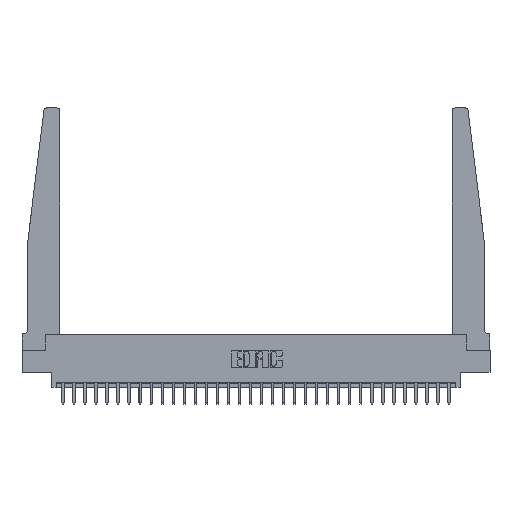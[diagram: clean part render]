
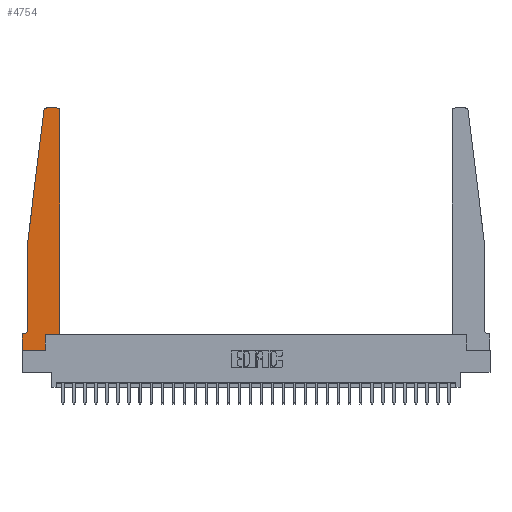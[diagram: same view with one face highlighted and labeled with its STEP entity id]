
A CAD part, top view. The second image highlights one B-rep face of the part: STEP entity #4754.
In plain terms, the highlighted planar face has unit normal (0, 0, 1).
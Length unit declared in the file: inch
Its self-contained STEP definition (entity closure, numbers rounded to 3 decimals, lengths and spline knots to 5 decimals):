
#468 = DIRECTION ( 'NONE',  ( 1., 0., 0. ) ) ;
#933 = CARTESIAN_POINT ( 'NONE',  ( 0., 0.1875, 0.37 ) ) ;
#1114 = DIRECTION ( 'NONE',  ( 0., -1., 0. ) ) ;
#1173 = VERTEX_POINT ( 'NONE', #16668 ) ;
#1797 = CARTESIAN_POINT ( 'NONE',  ( 0.015, 0.2375, 0.37 ) ) ;
#1874 = DIRECTION ( 'NONE',  ( 1., 0., 0. ) ) ;
#1889 = DIRECTION ( 'NONE',  ( 0., 0., 1. ) ) ;
#1945 = AXIS2_PLACEMENT_3D ( 'NONE', #16407, #14240, #468 ) ;
#2055 = DIRECTION ( 'NONE',  ( 0., 0., 1. ) ) ;
#2210 = CARTESIAN_POINT ( 'NONE',  ( 0.395, 2.72, 0.37 ) ) ;
#2400 = VERTEX_POINT ( 'NONE', #8629 ) ;
#2438 = DIRECTION ( 'NONE',  ( -0.122, -0.992, 0. ) ) ;
#2658 = ORIENTED_EDGE ( 'NONE', *, *, #6890, .T. ) ;
#2750 = VERTEX_POINT ( 'NONE', #17528 ) ;
#3119 = EDGE_CURVE ( 'NONE', #2400, #12083, #6324, .T. ) ;
#3208 = VECTOR ( 'NONE', #19406, 39.37008 ) ;
#4072 = DIRECTION ( 'NONE',  ( -1., 0., 0. ) ) ;
#4400 = VERTEX_POINT ( 'NONE', #13147 ) ;
#4754 = ADVANCED_FACE ( 'NONE', ( #12730 ), #25433, .T. ) ;
#5271 = CARTESIAN_POINT ( 'NONE',  ( 0.425, 0.18, 0.37 ) ) ;
#5695 = CARTESIAN_POINT ( 'NONE',  ( 0., 0., 0.37 ) ) ;
#6026 = EDGE_CURVE ( 'NONE', #26248, #22530, #23623, .T. ) ;
#6082 = CARTESIAN_POINT ( 'NONE',  ( 0.27653, 2.75, 0.37 ) ) ;
#6324 = CIRCLE ( 'NONE', #12543, 0.03 ) ;
#6637 = EDGE_CURVE ( 'NONE', #16781, #18427, #27081, .T. ) ;
#6890 = EDGE_CURVE ( 'NONE', #18427, #2750, #14757, .T. ) ;
#7164 = AXIS2_PLACEMENT_3D ( 'NONE', #1797, #17848, #4072 ) ;
#7378 = CARTESIAN_POINT ( 'NONE',  ( 0.2605, 0., 0.37 ) ) ;
#7553 = VERTEX_POINT ( 'NONE', #933 ) ;
#7600 = DIRECTION ( 'NONE',  ( 0., 1., 0. ) ) ;
#7764 = EDGE_CURVE ( 'NONE', #2750, #4400, #8866, .T. ) ;
#8091 = CARTESIAN_POINT ( 'NONE',  ( 0.395, 2.75, 0.37 ) ) ;
#8166 = EDGE_CURVE ( 'NONE', #22530, #2400, #22392, .T. ) ;
#8629 = CARTESIAN_POINT ( 'NONE',  ( 0.425, 2.72, 0.37 ) ) ;
#8652 = CARTESIAN_POINT ( 'NONE',  ( 0.065, 0.1875, 0.37 ) ) ;
#8866 = CIRCLE ( 'NONE', #7164, 0.05 ) ;
#9042 = LINE ( 'NONE', #13065, #25715 ) ;
#9522 = EDGE_CURVE ( 'NONE', #7553, #1173, #13518, .T. ) ;
#9527 = VECTOR ( 'NONE', #1114, 39.37008 ) ;
#9618 = DIRECTION ( 'NONE',  ( 1., 0., 0. ) ) ;
#10337 = EDGE_CURVE ( 'NONE', #1173, #13041, #28902, .T. ) ;
#10733 = DIRECTION ( 'NONE',  ( 0., 1., 0. ) ) ;
#10958 = DIRECTION ( 'NONE',  ( -1., 0., 0. ) ) ;
#11631 = EDGE_CURVE ( 'NONE', #13041, #26248, #9042, .T. ) ;
#12083 = VERTEX_POINT ( 'NONE', #8091 ) ;
#12296 = VECTOR ( 'NONE', #9618, 39.37008 ) ;
#12486 = ORIENTED_EDGE ( 'NONE', *, *, #6637, .T. ) ;
#12523 = CIRCLE ( 'NONE', #19577, 0.03 ) ;
#12543 = AXIS2_PLACEMENT_3D ( 'NONE', #2210, #2055, #1874 ) ;
#12699 = ORIENTED_EDGE ( 'NONE', *, *, #22779, .T. ) ;
#12730 = FACE_OUTER_BOUND ( 'NONE', #21836, .T. ) ;
#13041 = VERTEX_POINT ( 'NONE', #7378 ) ;
#13065 = CARTESIAN_POINT ( 'NONE',  ( 0.2605, 0.18, 0.37 ) ) ;
#13147 = CARTESIAN_POINT ( 'NONE',  ( 0.015, 0.1875, 0.37 ) ) ;
#13518 = LINE ( 'NONE', #5695, #9527 ) ;
#13965 = EDGE_CURVE ( 'NONE', #19576, #16781, #12523, .T. ) ;
#14240 = DIRECTION ( 'NONE',  ( 0., 0., 1. ) ) ;
#14418 = VECTOR ( 'NONE', #25931, 39.37008 ) ;
#14757 = LINE ( 'NONE', #17108, #3208 ) ;
#15323 = DIRECTION ( 'NONE',  ( 1., 0., 0. ) ) ;
#15574 = VECTOR ( 'NONE', #15323, 39.37008 ) ;
#15658 = CARTESIAN_POINT ( 'NONE',  ( 0.27653, 2.72, 0.37 ) ) ;
#16380 = VECTOR ( 'NONE', #7600, 39.37008 ) ;
#16407 = CARTESIAN_POINT ( 'NONE',  ( 0., 0.1875, 0.37 ) ) ;
#16426 = CARTESIAN_POINT ( 'NONE',  ( 0.24675, 2.72367, 0.37 ) ) ;
#16653 = ORIENTED_EDGE ( 'NONE', *, *, #13965, .T. ) ;
#16668 = CARTESIAN_POINT ( 'NONE',  ( 0., 0., 0.37 ) ) ;
#16781 = VERTEX_POINT ( 'NONE', #16426 ) ;
#16999 = VECTOR ( 'NONE', #10958, 39.37008 ) ;
#17108 = CARTESIAN_POINT ( 'NONE',  ( 0.065, 1.25, 0.37 ) ) ;
#17528 = CARTESIAN_POINT ( 'NONE',  ( 0.065, 0.2375, 0.37 ) ) ;
#17848 = DIRECTION ( 'NONE',  ( 0., 0., -1. ) ) ;
#17939 = DIRECTION ( 'NONE',  ( 1., 0., 0. ) ) ;
#18407 = CARTESIAN_POINT ( 'NONE',  ( 0.065, 1.25, 0.37 ) ) ;
#18427 = VERTEX_POINT ( 'NONE', #19705 ) ;
#19290 = CARTESIAN_POINT ( 'NONE',  ( 0.2605, 0.18, 0.37 ) ) ;
#19406 = DIRECTION ( 'NONE',  ( 0., -1., 0. ) ) ;
#19576 = VERTEX_POINT ( 'NONE', #6082 ) ;
#19577 = AXIS2_PLACEMENT_3D ( 'NONE', #15658, #1889, #17939 ) ;
#19705 = CARTESIAN_POINT ( 'NONE',  ( 0.065, 1.25, 0.37 ) ) ;
#20669 = CARTESIAN_POINT ( 'NONE',  ( 0.425, 0.18, 0.37 ) ) ;
#20981 = EDGE_CURVE ( 'NONE', #4400, #7553, #22979, .T. ) ;
#21836 = EDGE_LOOP ( 'NONE', ( #12699, #16653, #12486, #2658, #27409, #27586, #27639, #28007, #28129, #28249, #28636, #28694 ) ) ;
#22392 = LINE ( 'NONE', #5271, #16380 ) ;
#22530 = VERTEX_POINT ( 'NONE', #20669 ) ;
#22779 = EDGE_CURVE ( 'NONE', #12083, #19576, #24968, .T. ) ;
#22979 = LINE ( 'NONE', #8652, #16999 ) ;
#23623 = LINE ( 'NONE', #25477, #12296 ) ;
#23672 = CARTESIAN_POINT ( 'NONE',  ( 0.25, 2.75, 0.37 ) ) ;
#24282 = CARTESIAN_POINT ( 'NONE',  ( 0., 0., 0.37 ) ) ;
#24968 = LINE ( 'NONE', #23672, #14418 ) ;
#25433 = PLANE ( 'NONE',  #1945 ) ;
#25477 = CARTESIAN_POINT ( 'NONE',  ( 0.425, 0.18, 0.37 ) ) ;
#25715 = VECTOR ( 'NONE', #10733, 39.37008 ) ;
#25931 = DIRECTION ( 'NONE',  ( -1., 0., 0. ) ) ;
#26248 = VERTEX_POINT ( 'NONE', #19290 ) ;
#26388 = VECTOR ( 'NONE', #2438, 39.37008 ) ;
#27081 = LINE ( 'NONE', #18407, #26388 ) ;
#27409 = ORIENTED_EDGE ( 'NONE', *, *, #7764, .T. ) ;
#27586 = ORIENTED_EDGE ( 'NONE', *, *, #20981, .T. ) ;
#27639 = ORIENTED_EDGE ( 'NONE', *, *, #9522, .T. ) ;
#28007 = ORIENTED_EDGE ( 'NONE', *, *, #10337, .T. ) ;
#28129 = ORIENTED_EDGE ( 'NONE', *, *, #11631, .T. ) ;
#28249 = ORIENTED_EDGE ( 'NONE', *, *, #6026, .T. ) ;
#28636 = ORIENTED_EDGE ( 'NONE', *, *, #8166, .T. ) ;
#28694 = ORIENTED_EDGE ( 'NONE', *, *, #3119, .T. ) ;
#28902 = LINE ( 'NONE', #24282, #15574 ) ;
